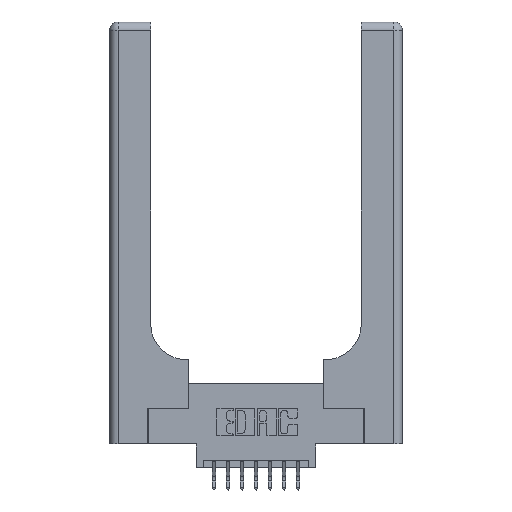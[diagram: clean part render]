
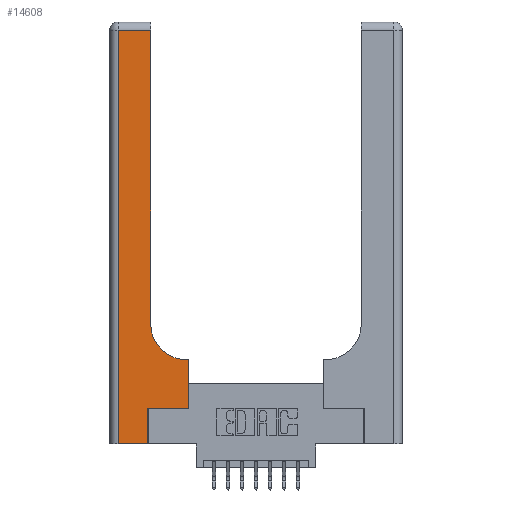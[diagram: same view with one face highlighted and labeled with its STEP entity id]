
A CAD part, top view. The second image highlights one B-rep face of the part: STEP entity #14608.
In plain terms, the highlighted planar face has unit normal (0, 0, 1).
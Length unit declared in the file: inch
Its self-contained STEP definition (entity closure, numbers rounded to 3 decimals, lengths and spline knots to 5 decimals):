
#37 = EDGE_CURVE ( 'NONE', #8700, #1182, #14993, .T. ) ;
#38 = VERTEX_POINT ( 'NONE', #12495 ) ;
#156 = CARTESIAN_POINT ( 'NONE',  ( 0.269, 0.25, 0.37 ) ) ;
#158 = EDGE_CURVE ( 'NONE', #1066, #38, #10402, .T. ) ;
#264 = ORIENTED_EDGE ( 'NONE', *, *, #37, .T. ) ;
#386 = LINE ( 'NONE', #1402, #6671 ) ;
#405 = PLANE ( 'NONE',  #8475 ) ;
#440 = ORIENTED_EDGE ( 'NONE', *, *, #13828, .T. ) ;
#634 = VERTEX_POINT ( 'NONE', #9600 ) ;
#651 = EDGE_CURVE ( 'NONE', #38, #14979, #8319, .T. ) ;
#1035 = CARTESIAN_POINT ( 'NONE',  ( 0.5415, 0.6, 0.37 ) ) ;
#1066 = VERTEX_POINT ( 'NONE', #1035 ) ;
#1130 = VERTEX_POINT ( 'NONE', #156 ) ;
#1182 = VERTEX_POINT ( 'NONE', #6843 ) ;
#1402 = CARTESIAN_POINT ( 'NONE',  ( 0., 0., 0.37 ) ) ;
#1414 = VECTOR ( 'NONE', #11049, 39.37008 ) ;
#2871 = CARTESIAN_POINT ( 'NONE',  ( 0.269, 0., 0.37 ) ) ;
#3585 = VERTEX_POINT ( 'NONE', #14815 ) ;
#4226 = DIRECTION ( 'NONE',  ( -1., 0., 0. ) ) ;
#5340 = CARTESIAN_POINT ( 'NONE',  ( 0., 2.94, 0.37 ) ) ;
#5437 = ORIENTED_EDGE ( 'NONE', *, *, #11796, .T. ) ;
#5647 = LINE ( 'NONE', #6194, #11665 ) ;
#5822 = EDGE_CURVE ( 'NONE', #1182, #1066, #13095, .T. ) ;
#5985 = CARTESIAN_POINT ( 'NONE',  ( 0.2915, 2.94, 0.37 ) ) ;
#6117 = CARTESIAN_POINT ( 'NONE',  ( 0.2915, 0.6, 0.37 ) ) ;
#6194 = CARTESIAN_POINT ( 'NONE',  ( 0.269, 0.25, 0.37 ) ) ;
#6356 = VECTOR ( 'NONE', #13289, 39.37008 ) ;
#6645 = VERTEX_POINT ( 'NONE', #2871 ) ;
#6671 = VECTOR ( 'NONE', #7574, 39.37008 ) ;
#6843 = CARTESIAN_POINT ( 'NONE',  ( 0.5585, 0.6, 0.37 ) ) ;
#7036 = AXIS2_PLACEMENT_3D ( 'NONE', #7396, #7360, #7340 ) ;
#7113 = ORIENTED_EDGE ( 'NONE', *, *, #14543, .T. ) ;
#7340 = DIRECTION ( 'NONE',  ( 1., 0., 0. ) ) ;
#7360 = DIRECTION ( 'NONE',  ( 0., 0., -1. ) ) ;
#7396 = CARTESIAN_POINT ( 'NONE',  ( 0.5415, 0.85, 0.37 ) ) ;
#7431 = DIRECTION ( 'NONE',  ( 1., 0., 0. ) ) ;
#7574 = DIRECTION ( 'NONE',  ( 1., 0., 0. ) ) ;
#7608 = LINE ( 'NONE', #9876, #1414 ) ;
#7615 = DIRECTION ( 'NONE',  ( 0., -1., 0. ) ) ;
#8239 = EDGE_CURVE ( 'NONE', #634, #6645, #386, .T. ) ;
#8319 = LINE ( 'NONE', #9380, #14255 ) ;
#8475 = AXIS2_PLACEMENT_3D ( 'NONE', #13807, #11489, #4226 ) ;
#8700 = VERTEX_POINT ( 'NONE', #11124 ) ;
#9344 = DIRECTION ( 'NONE',  ( 0., 1., 0. ) ) ;
#9380 = CARTESIAN_POINT ( 'NONE',  ( 0.2915, 3., 0.37 ) ) ;
#9600 = CARTESIAN_POINT ( 'NONE',  ( 0.06, 0., 0.37 ) ) ;
#9708 = ORIENTED_EDGE ( 'NONE', *, *, #158, .T. ) ;
#9876 = CARTESIAN_POINT ( 'NONE',  ( 0.269, 0., 0.37 ) ) ;
#10207 = DIRECTION ( 'NONE',  ( -1., 0., 0. ) ) ;
#10350 = FACE_OUTER_BOUND ( 'NONE', #14286, .T. ) ;
#10402 = CIRCLE ( 'NONE', #7036, 0.25 ) ;
#10419 = ORIENTED_EDGE ( 'NONE', *, *, #651, .T. ) ;
#10641 = ORIENTED_EDGE ( 'NONE', *, *, #14453, .T. ) ;
#10727 = LINE ( 'NONE', #5340, #13850 ) ;
#11049 = DIRECTION ( 'NONE',  ( 0., 1., 0. ) ) ;
#11124 = CARTESIAN_POINT ( 'NONE',  ( 0.5585, 0.25, 0.37 ) ) ;
#11489 = DIRECTION ( 'NONE',  ( 0., 0., -1. ) ) ;
#11665 = VECTOR ( 'NONE', #7431, 39.37008 ) ;
#11796 = EDGE_CURVE ( 'NONE', #6645, #1130, #7608, .T. ) ;
#12372 = CARTESIAN_POINT ( 'NONE',  ( 0.06, 3., 0.37 ) ) ;
#12495 = CARTESIAN_POINT ( 'NONE',  ( 0.2915, 0.85, 0.37 ) ) ;
#12645 = DIRECTION ( 'NONE',  ( 0., 1., 0. ) ) ;
#13053 = ORIENTED_EDGE ( 'NONE', *, *, #8239, .T. ) ;
#13095 = LINE ( 'NONE', #6117, #6356 ) ;
#13289 = DIRECTION ( 'NONE',  ( -1., 0., 0. ) ) ;
#13732 = CARTESIAN_POINT ( 'NONE',  ( 0.5585, 0.25, 0.37 ) ) ;
#13807 = CARTESIAN_POINT ( 'NONE',  ( 0., 3., 0.37 ) ) ;
#13828 = EDGE_CURVE ( 'NONE', #1130, #8700, #5647, .T. ) ;
#13850 = VECTOR ( 'NONE', #10207, 39.37008 ) ;
#14028 = ORIENTED_EDGE ( 'NONE', *, *, #5822, .T. ) ;
#14255 = VECTOR ( 'NONE', #9344, 39.37008 ) ;
#14286 = EDGE_LOOP ( 'NONE', ( #10419, #7113, #10641, #13053, #5437, #440, #264, #14028, #9708 ) ) ;
#14453 = EDGE_CURVE ( 'NONE', #3585, #634, #15309, .T. ) ;
#14543 = EDGE_CURVE ( 'NONE', #14979, #3585, #10727, .T. ) ;
#14608 = ADVANCED_FACE ( 'NONE', ( #10350 ), #405, .F. ) ;
#14627 = VECTOR ( 'NONE', #12645, 39.37008 ) ;
#14815 = CARTESIAN_POINT ( 'NONE',  ( 0.06, 2.94, 0.37 ) ) ;
#14945 = VECTOR ( 'NONE', #7615, 39.37008 ) ;
#14979 = VERTEX_POINT ( 'NONE', #5985 ) ;
#14993 = LINE ( 'NONE', #13732, #14627 ) ;
#15309 = LINE ( 'NONE', #12372, #14945 ) ;
